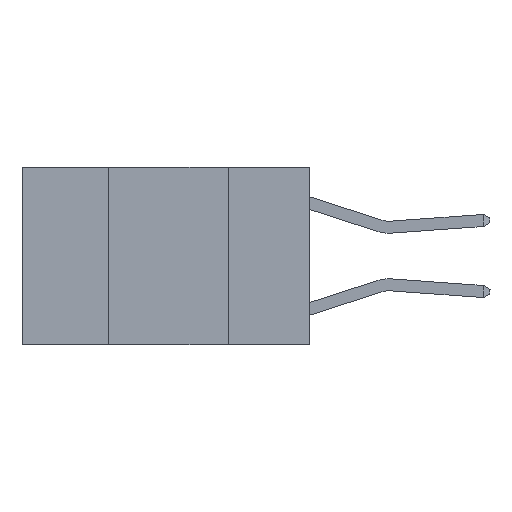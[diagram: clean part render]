
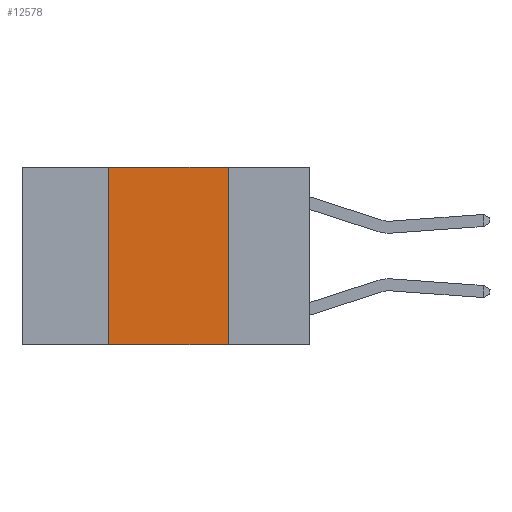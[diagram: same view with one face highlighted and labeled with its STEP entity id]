
A CAD part, left-side view. The second image highlights one B-rep face of the part: STEP entity #12578.
In plain terms, the highlighted planar face has unit normal (-1, 0, 0).
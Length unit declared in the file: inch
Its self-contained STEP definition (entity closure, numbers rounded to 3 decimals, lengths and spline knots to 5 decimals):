
#105 = LINE ( 'NONE', #11336, #5074 ) ;
#584 = EDGE_CURVE ( 'NONE', #9609, #11350, #2107, .T. ) ;
#628 = LINE ( 'NONE', #3848, #10727 ) ;
#1618 = DIRECTION ( 'NONE',  ( 0., 0., 1. ) ) ;
#1670 = DIRECTION ( 'NONE',  ( 0., -1., 0. ) ) ;
#1695 = EDGE_CURVE ( 'NONE', #2555, #11350, #628, .T. ) ;
#1795 = VECTOR ( 'NONE', #3011, 39.37008 ) ;
#2107 = LINE ( 'NONE', #3542, #1795 ) ;
#2555 = VERTEX_POINT ( 'NONE', #12428 ) ;
#2632 = CARTESIAN_POINT ( 'NONE',  ( 0., 0.42, 0. ) ) ;
#2951 = VERTEX_POINT ( 'NONE', #9550 ) ;
#3011 = DIRECTION ( 'NONE',  ( 0., -1., 0. ) ) ;
#3542 = CARTESIAN_POINT ( 'NONE',  ( 0., 0.6, -0.37 ) ) ;
#3651 = CARTESIAN_POINT ( 'NONE',  ( 0., 0.6, 0. ) ) ;
#3848 = CARTESIAN_POINT ( 'NONE',  ( 0., 0.17, 0. ) ) ;
#3851 = EDGE_CURVE ( 'NONE', #2951, #2555, #105, .T. ) ;
#4624 = DIRECTION ( 'NONE',  ( 1., 0., 0. ) ) ;
#5074 = VECTOR ( 'NONE', #1670, 39.37008 ) ;
#5796 = VECTOR ( 'NONE', #1618, 39.37008 ) ;
#6533 = EDGE_CURVE ( 'NONE', #9609, #2951, #11209, .T. ) ;
#7386 = ORIENTED_EDGE ( 'NONE', *, *, #584, .T. ) ;
#7604 = AXIS2_PLACEMENT_3D ( 'NONE', #3651, #4624, #11340 ) ;
#8200 = ORIENTED_EDGE ( 'NONE', *, *, #1695, .F. ) ;
#8647 = DIRECTION ( 'NONE',  ( 0., 0., -1. ) ) ;
#8965 = EDGE_LOOP ( 'NONE', ( #8200, #11540, #10416, #7386 ) ) ;
#9403 = PLANE ( 'NONE',  #7604 ) ;
#9550 = CARTESIAN_POINT ( 'NONE',  ( 0., 0.42, 0. ) ) ;
#9609 = VERTEX_POINT ( 'NONE', #9684 ) ;
#9684 = CARTESIAN_POINT ( 'NONE',  ( 0., 0.42, -0.37 ) ) ;
#10008 = FACE_OUTER_BOUND ( 'NONE', #8965, .T. ) ;
#10416 = ORIENTED_EDGE ( 'NONE', *, *, #6533, .F. ) ;
#10727 = VECTOR ( 'NONE', #8647, 39.37008 ) ;
#11209 = LINE ( 'NONE', #2632, #5796 ) ;
#11336 = CARTESIAN_POINT ( 'NONE',  ( 0., 0.6, 0. ) ) ;
#11340 = DIRECTION ( 'NONE',  ( 0., 0., -1. ) ) ;
#11350 = VERTEX_POINT ( 'NONE', #12367 ) ;
#11540 = ORIENTED_EDGE ( 'NONE', *, *, #3851, .F. ) ;
#12367 = CARTESIAN_POINT ( 'NONE',  ( 0., 0.17, -0.37 ) ) ;
#12428 = CARTESIAN_POINT ( 'NONE',  ( 0., 0.17, 0. ) ) ;
#12578 = ADVANCED_FACE ( 'NONE', ( #10008 ), #9403, .F. ) ;
